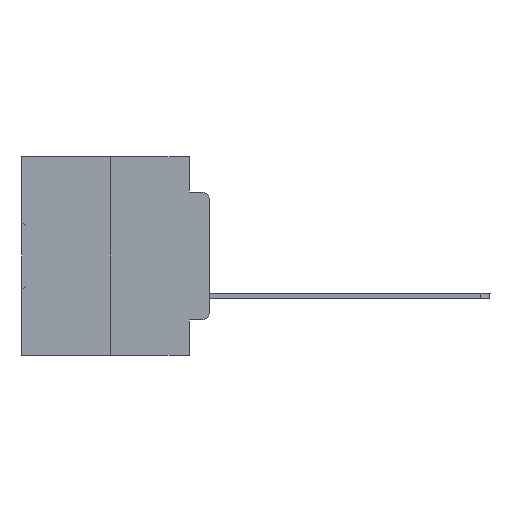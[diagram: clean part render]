
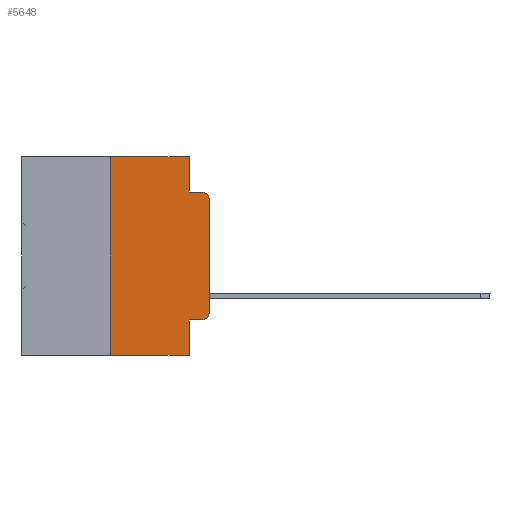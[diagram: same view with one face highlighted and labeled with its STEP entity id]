
A CAD part, left-side view. The second image highlights one B-rep face of the part: STEP entity #5648.
In plain terms, the highlighted planar face has unit normal (-1, 0, 0).
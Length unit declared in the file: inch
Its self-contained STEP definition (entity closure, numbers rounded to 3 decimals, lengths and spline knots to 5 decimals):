
#441 = LINE ( 'NONE', #27648, #23310 ) ;
#1248 = ORIENTED_EDGE ( 'NONE', *, *, #32135, .T. ) ;
#1424 = VERTEX_POINT ( 'NONE', #27285 ) ;
#1742 = EDGE_LOOP ( 'NONE', ( #1248, #28697, #24672, #16841, #5392, #20757, #28182, #3265, #6989, #9584 ) ) ;
#2860 = DIRECTION ( 'NONE',  ( 0., -1., 0. ) ) ;
#3109 = CARTESIAN_POINT ( 'NONE',  ( 0., 0.473, 0. ) ) ;
#3265 = ORIENTED_EDGE ( 'NONE', *, *, #13020, .F. ) ;
#3452 = VERTEX_POINT ( 'NONE', #16668 ) ;
#3531 = CARTESIAN_POINT ( 'NONE',  ( 0., 0.25, 0. ) ) ;
#3604 = LINE ( 'NONE', #23352, #27731 ) ;
#5299 = DIRECTION ( 'NONE',  ( 0., 0., -1. ) ) ;
#5346 = DIRECTION ( 'NONE',  ( 1., 0., 0. ) ) ;
#5392 = ORIENTED_EDGE ( 'NONE', *, *, #28267, .F. ) ;
#5570 = EDGE_CURVE ( 'NONE', #17860, #10611, #31094, .T. ) ;
#5648 = ADVANCED_FACE ( 'NONE', ( #7889 ), #30583, .F. ) ;
#5675 = DIRECTION ( 'NONE',  ( 0., 0., -1. ) ) ;
#5828 = VECTOR ( 'NONE', #14065, 39.37008 ) ;
#5917 = EDGE_CURVE ( 'NONE', #22990, #3452, #11290, .T. ) ;
#5985 = VECTOR ( 'NONE', #5299, 39.37008 ) ;
#6113 = EDGE_CURVE ( 'NONE', #19161, #9006, #441, .T. ) ;
#6398 = LINE ( 'NONE', #32264, #5985 ) ;
#6989 = ORIENTED_EDGE ( 'NONE', *, *, #5570, .T. ) ;
#7399 = CARTESIAN_POINT ( 'NONE',  ( 0., 0.25, 0. ) ) ;
#7733 = DIRECTION ( 'NONE',  ( 0., 0., -1. ) ) ;
#7889 = FACE_OUTER_BOUND ( 'NONE', #1742, .T. ) ;
#8069 = AXIS2_PLACEMENT_3D ( 'NONE', #3109, #5346, #5675 ) ;
#8814 = CARTESIAN_POINT ( 'NONE',  ( 0., 0., -0.1085 ) ) ;
#8929 = VERTEX_POINT ( 'NONE', #30527 ) ;
#9006 = VERTEX_POINT ( 'NONE', #28298 ) ;
#9358 = EDGE_CURVE ( 'NONE', #8929, #32758, #3604, .T. ) ;
#9584 = ORIENTED_EDGE ( 'NONE', *, *, #13027, .T. ) ;
#10611 = VERTEX_POINT ( 'NONE', #13916 ) ;
#11290 = CIRCLE ( 'NONE', #30389, 0.02 ) ;
#12658 = CARTESIAN_POINT ( 'NONE',  ( 0., 0.051, -0.4115 ) ) ;
#12905 = CARTESIAN_POINT ( 'NONE',  ( 0., 0.051, -0.0885 ) ) ;
#12951 = LINE ( 'NONE', #12905, #13816 ) ;
#13020 = EDGE_CURVE ( 'NONE', #17860, #9006, #6398, .T. ) ;
#13027 = EDGE_CURVE ( 'NONE', #10611, #1424, #34433, .T. ) ;
#13661 = EDGE_CURVE ( 'NONE', #32758, #3452, #12951, .T. ) ;
#13816 = VECTOR ( 'NONE', #29140, 39.37008 ) ;
#13916 = CARTESIAN_POINT ( 'NONE',  ( 0., 0.02, -0.4115 ) ) ;
#14065 = DIRECTION ( 'NONE',  ( 0., 0., 1. ) ) ;
#14708 = DIRECTION ( 'NONE',  ( 0., -1., 0. ) ) ;
#14723 = LINE ( 'NONE', #24649, #23790 ) ;
#15842 = CARTESIAN_POINT ( 'NONE',  ( 0., 0.051, -0.4115 ) ) ;
#16668 = CARTESIAN_POINT ( 'NONE',  ( 0., 0.02, -0.0885 ) ) ;
#16841 = ORIENTED_EDGE ( 'NONE', *, *, #9358, .F. ) ;
#17860 = VERTEX_POINT ( 'NONE', #12658 ) ;
#18180 = DIRECTION ( 'NONE',  ( 0., 0., -1. ) ) ;
#19161 = VERTEX_POINT ( 'NONE', #22210 ) ;
#19306 = CARTESIAN_POINT ( 'NONE',  ( 0., 0.051, -0.0885 ) ) ;
#20477 = LINE ( 'NONE', #3531, #5828 ) ;
#20757 = ORIENTED_EDGE ( 'NONE', *, *, #25508, .F. ) ;
#22210 = CARTESIAN_POINT ( 'NONE',  ( 0., 0.25, -0.5 ) ) ;
#22990 = VERTEX_POINT ( 'NONE', #8814 ) ;
#23310 = VECTOR ( 'NONE', #2860, 39.37008 ) ;
#23352 = CARTESIAN_POINT ( 'NONE',  ( 0., 0.051, 0. ) ) ;
#23790 = VECTOR ( 'NONE', #24985, 39.37008 ) ;
#23945 = LINE ( 'NONE', #31670, #27379 ) ;
#24195 = DIRECTION ( 'NONE',  ( -1., 0., 0. ) ) ;
#24649 = CARTESIAN_POINT ( 'NONE',  ( 0., 0., 0. ) ) ;
#24672 = ORIENTED_EDGE ( 'NONE', *, *, #13661, .F. ) ;
#24985 = DIRECTION ( 'NONE',  ( 0., 0., 1. ) ) ;
#25508 = EDGE_CURVE ( 'NONE', #19161, #26168, #20477, .T. ) ;
#25930 = VECTOR ( 'NONE', #33350, 39.37008 ) ;
#26168 = VERTEX_POINT ( 'NONE', #7399 ) ;
#26834 = DIRECTION ( 'NONE',  ( 0., 0., -1. ) ) ;
#27063 = CARTESIAN_POINT ( 'NONE',  ( 0., 0.02, -0.3915 ) ) ;
#27285 = CARTESIAN_POINT ( 'NONE',  ( 0., 0., -0.3915 ) ) ;
#27323 = CARTESIAN_POINT ( 'NONE',  ( 0., 0.02, -0.1085 ) ) ;
#27379 = VECTOR ( 'NONE', #14708, 39.37008 ) ;
#27648 = CARTESIAN_POINT ( 'NONE',  ( 0., 0.473, -0.5 ) ) ;
#27731 = VECTOR ( 'NONE', #18180, 39.37008 ) ;
#28182 = ORIENTED_EDGE ( 'NONE', *, *, #6113, .T. ) ;
#28267 = EDGE_CURVE ( 'NONE', #26168, #8929, #23945, .T. ) ;
#28298 = CARTESIAN_POINT ( 'NONE',  ( 0., 0.051, -0.5 ) ) ;
#28697 = ORIENTED_EDGE ( 'NONE', *, *, #5917, .T. ) ;
#29140 = DIRECTION ( 'NONE',  ( 0., -1., 0. ) ) ;
#30389 = AXIS2_PLACEMENT_3D ( 'NONE', #27323, #35158, #7733 ) ;
#30527 = CARTESIAN_POINT ( 'NONE',  ( 0., 0.051, 0. ) ) ;
#30583 = PLANE ( 'NONE',  #8069 ) ;
#31094 = LINE ( 'NONE', #15842, #25930 ) ;
#31670 = CARTESIAN_POINT ( 'NONE',  ( 0., 0.473, 0. ) ) ;
#32135 = EDGE_CURVE ( 'NONE', #1424, #22990, #14723, .T. ) ;
#32264 = CARTESIAN_POINT ( 'NONE',  ( 0., 0.051, 0. ) ) ;
#32758 = VERTEX_POINT ( 'NONE', #19306 ) ;
#33350 = DIRECTION ( 'NONE',  ( 0., -1., 0. ) ) ;
#34272 = AXIS2_PLACEMENT_3D ( 'NONE', #27063, #24195, #26834 ) ;
#34433 = CIRCLE ( 'NONE', #34272, 0.02 ) ;
#35158 = DIRECTION ( 'NONE',  ( -1., 0., 0. ) ) ;
